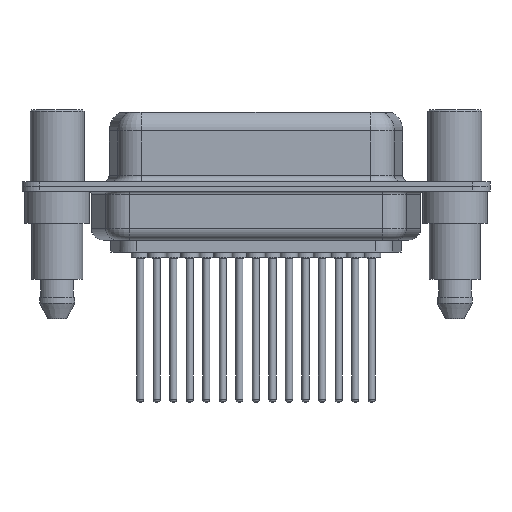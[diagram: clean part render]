
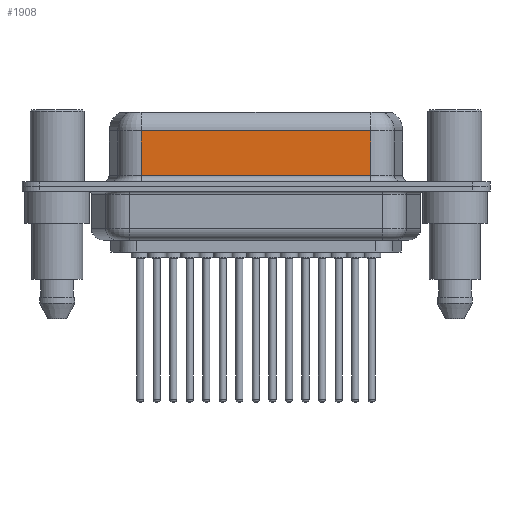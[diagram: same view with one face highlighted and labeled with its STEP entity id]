
A CAD part, front view. The second image highlights one B-rep face of the part: STEP entity #1908.
In plain terms, the highlighted planar face has unit normal (0, -1, 0).
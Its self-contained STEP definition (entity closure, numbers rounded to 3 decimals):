
#91 = LINE ( 'NONE', #11073, #1201 ) ;
#327 = CARTESIAN_POINT ( 'NONE',  ( 26.262, -3.95, 6.4 ) ) ;
#1015 = CARTESIAN_POINT ( 'NONE',  ( 26.262, -3.95, 0.9 ) ) ;
#1201 = VECTOR ( 'NONE', #18198, 1000. ) ;
#1908 = ADVANCED_FACE ( 'NONE', ( #5467 ), #2556, .F. ) ;
#2358 = VECTOR ( 'NONE', #15155, 1000. ) ;
#2556 = PLANE ( 'NONE',  #6601 ) ;
#2706 = CARTESIAN_POINT ( 'NONE',  ( 7.038, -3.95, 0.9 ) ) ;
#3354 = VERTEX_POINT ( 'NONE', #16673 ) ;
#5329 = ORIENTED_EDGE ( 'NONE', *, *, #10988, .T. ) ;
#5467 = FACE_OUTER_BOUND ( 'NONE', #14459, .T. ) ;
#6100 = VECTOR ( 'NONE', #15930, 1000. ) ;
#6601 = AXIS2_PLACEMENT_3D ( 'NONE', #10540, #12546, #14799 ) ;
#6690 = VERTEX_POINT ( 'NONE', #2706 ) ;
#6779 = EDGE_CURVE ( 'NONE', #11172, #3354, #7364, .T. ) ;
#7089 = EDGE_CURVE ( 'NONE', #11172, #13624, #16569, .T. ) ;
#7364 = LINE ( 'NONE', #327, #6100 ) ;
#10519 = VECTOR ( 'NONE', #14319, 1000. ) ;
#10540 = CARTESIAN_POINT ( 'NONE',  ( 26.262, -3.95, 6.4 ) ) ;
#10988 = EDGE_CURVE ( 'NONE', #13624, #6690, #91, .T. ) ;
#11073 = CARTESIAN_POINT ( 'NONE',  ( 7.038, -3.95, 6.4 ) ) ;
#11172 = VERTEX_POINT ( 'NONE', #12924 ) ;
#11349 = ORIENTED_EDGE ( 'NONE', *, *, #6779, .F. ) ;
#11874 = ORIENTED_EDGE ( 'NONE', *, *, #12921, .T. ) ;
#12546 = DIRECTION ( 'NONE',  ( 0., 1., 0. ) ) ;
#12921 = EDGE_CURVE ( 'NONE', #6690, #3354, #13665, .T. ) ;
#12924 = CARTESIAN_POINT ( 'NONE',  ( 26.262, -3.95, 4.65 ) ) ;
#13624 = VERTEX_POINT ( 'NONE', #13809 ) ;
#13665 = LINE ( 'NONE', #1015, #2358 ) ;
#13780 = ORIENTED_EDGE ( 'NONE', *, *, #7089, .T. ) ;
#13796 = CARTESIAN_POINT ( 'NONE',  ( 26.262, -3.95, 4.65 ) ) ;
#13809 = CARTESIAN_POINT ( 'NONE',  ( 7.038, -3.95, 4.65 ) ) ;
#14319 = DIRECTION ( 'NONE',  ( -1., 0., 0. ) ) ;
#14459 = EDGE_LOOP ( 'NONE', ( #11349, #13780, #5329, #11874 ) ) ;
#14799 = DIRECTION ( 'NONE',  ( -1., 0., 0. ) ) ;
#15155 = DIRECTION ( 'NONE',  ( 1., 0., 0. ) ) ;
#15930 = DIRECTION ( 'NONE',  ( 0., 0., -1. ) ) ;
#16569 = LINE ( 'NONE', #13796, #10519 ) ;
#16673 = CARTESIAN_POINT ( 'NONE',  ( 26.262, -3.95, 0.9 ) ) ;
#18198 = DIRECTION ( 'NONE',  ( 0., 0., -1. ) ) ;
